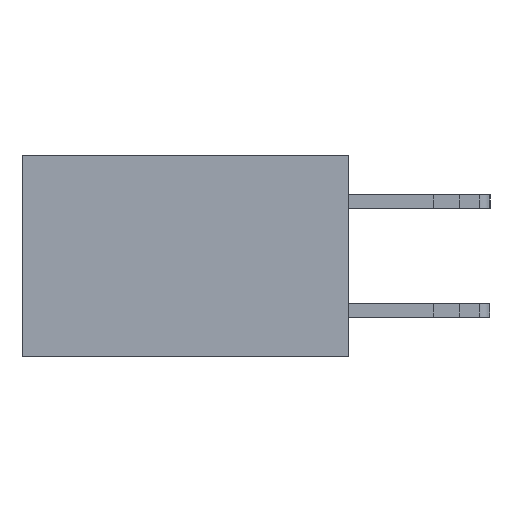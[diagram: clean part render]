
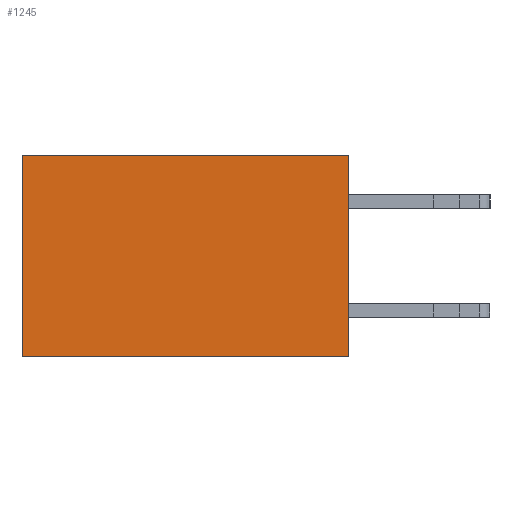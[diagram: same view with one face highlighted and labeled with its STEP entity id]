
A CAD part, left-side view. The second image highlights one B-rep face of the part: STEP entity #1245.
In plain terms, the highlighted planar face has unit normal (-1, 0, 0).
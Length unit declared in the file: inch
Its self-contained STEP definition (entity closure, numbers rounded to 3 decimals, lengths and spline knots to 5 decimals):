
#156 = CARTESIAN_POINT ( 'NONE',  ( 0.298, 0., 0. ) ) ;
#513 = FACE_OUTER_BOUND ( 'NONE', #4474, .T. ) ;
#1245 = ADVANCED_FACE ( 'NONE', ( #513 ), #3304, .F. ) ;
#1401 = CARTESIAN_POINT ( 'NONE',  ( 0.298, 0., -0.37 ) ) ;
#2103 = LINE ( 'NONE', #156, #14645 ) ;
#3304 = PLANE ( 'NONE',  #10037 ) ;
#3688 = ORIENTED_EDGE ( 'NONE', *, *, #6116, .T. ) ;
#4316 = VERTEX_POINT ( 'NONE', #8999 ) ;
#4474 = EDGE_LOOP ( 'NONE', ( #3688, #8057, #4523, #15123 ) ) ;
#4523 = ORIENTED_EDGE ( 'NONE', *, *, #5118, .F. ) ;
#4527 = CARTESIAN_POINT ( 'NONE',  ( 0.298, 0., 0. ) ) ;
#4540 = VERTEX_POINT ( 'NONE', #5855 ) ;
#5118 = EDGE_CURVE ( 'NONE', #10846, #4540, #7291, .T. ) ;
#5855 = CARTESIAN_POINT ( 'NONE',  ( 0.298, 0., -0.37 ) ) ;
#6116 = EDGE_CURVE ( 'NONE', #4316, #16256, #8929, .T. ) ;
#6253 = DIRECTION ( 'NONE',  ( 0., 1., 0. ) ) ;
#7291 = LINE ( 'NONE', #8812, #10432 ) ;
#8057 = ORIENTED_EDGE ( 'NONE', *, *, #12418, .F. ) ;
#8128 = DIRECTION ( 'NONE',  ( 0., 0., -1. ) ) ;
#8171 = CARTESIAN_POINT ( 'NONE',  ( 0.298, 0.6, 0. ) ) ;
#8340 = EDGE_CURVE ( 'NONE', #10846, #4316, #2103, .T. ) ;
#8435 = LINE ( 'NONE', #1401, #12387 ) ;
#8812 = CARTESIAN_POINT ( 'NONE',  ( 0.298, 0., 0. ) ) ;
#8929 = LINE ( 'NONE', #8171, #15363 ) ;
#8999 = CARTESIAN_POINT ( 'NONE',  ( 0.298, 0.6, 0. ) ) ;
#9391 = DIRECTION ( 'NONE',  ( 0., 0., -1. ) ) ;
#9674 = CARTESIAN_POINT ( 'NONE',  ( 0.298, 0.6, -0.37 ) ) ;
#10037 = AXIS2_PLACEMENT_3D ( 'NONE', #13030, #10627, #12909 ) ;
#10432 = VECTOR ( 'NONE', #9391, 39.37008 ) ;
#10627 = DIRECTION ( 'NONE',  ( 1., 0., 0. ) ) ;
#10846 = VERTEX_POINT ( 'NONE', #4527 ) ;
#12387 = VECTOR ( 'NONE', #15584, 39.37008 ) ;
#12418 = EDGE_CURVE ( 'NONE', #4540, #16256, #8435, .T. ) ;
#12909 = DIRECTION ( 'NONE',  ( 0., 0., -1. ) ) ;
#13030 = CARTESIAN_POINT ( 'NONE',  ( 0.298, 0., 0. ) ) ;
#14645 = VECTOR ( 'NONE', #6253, 39.37008 ) ;
#15123 = ORIENTED_EDGE ( 'NONE', *, *, #8340, .T. ) ;
#15363 = VECTOR ( 'NONE', #8128, 39.37008 ) ;
#15584 = DIRECTION ( 'NONE',  ( 0., 1., 0. ) ) ;
#16256 = VERTEX_POINT ( 'NONE', #9674 ) ;
